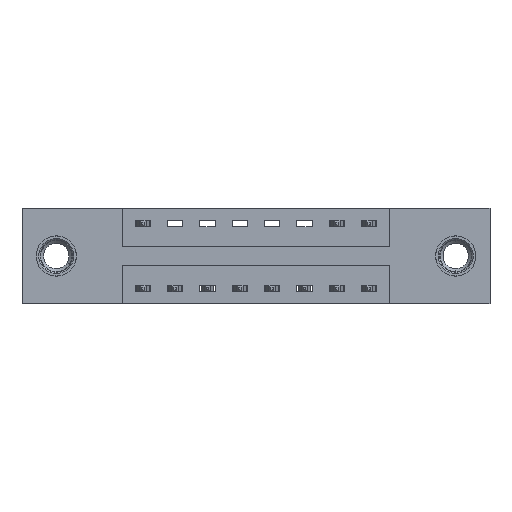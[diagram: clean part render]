
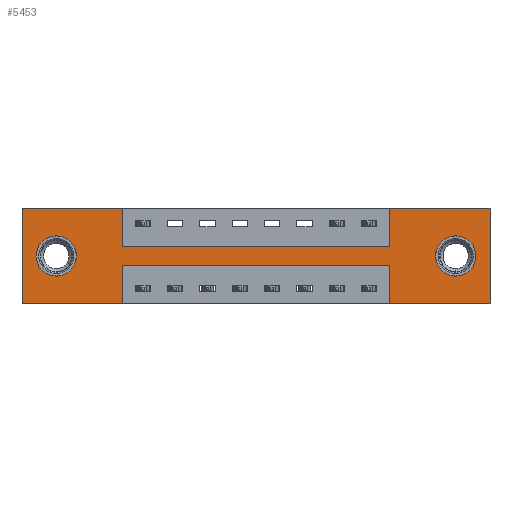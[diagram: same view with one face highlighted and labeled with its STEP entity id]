
A CAD part, front view. The second image highlights one B-rep face of the part: STEP entity #5453.
In plain terms, the highlighted planar face has unit normal (0, -1, 0).
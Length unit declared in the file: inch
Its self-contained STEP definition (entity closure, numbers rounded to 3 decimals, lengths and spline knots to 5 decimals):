
#43 = DIRECTION ( 'NONE',  ( 0., 0., 1. ) ) ;
#82 = VECTOR ( 'NONE', #8620, 39.37008 ) ;
#323 = EDGE_CURVE ( 'NONE', #2774, #729, #4343, .T. ) ;
#348 = CARTESIAN_POINT ( 'NONE',  ( 0., 0., 0. ) ) ;
#426 = DIRECTION ( 'NONE',  ( -1., 0., 0. ) ) ;
#499 = ORIENTED_EDGE ( 'NONE', *, *, #1237, .F. ) ;
#500 = CARTESIAN_POINT ( 'NONE',  ( 1.6775, 0., -0.107 ) ) ;
#535 = CARTESIAN_POINT ( 'NONE',  ( 0., 0., -0.37 ) ) ;
#729 = VERTEX_POINT ( 'NONE', #921 ) ;
#777 = VECTOR ( 'NONE', #8164, 39.37008 ) ;
#783 = ORIENTED_EDGE ( 'NONE', *, *, #1724, .F. ) ;
#921 = CARTESIAN_POINT ( 'NONE',  ( 0.3875, 0., -0.15 ) ) ;
#1048 = ORIENTED_EDGE ( 'NONE', *, *, #2806, .F. ) ;
#1144 = LINE ( 'NONE', #5271, #7589 ) ;
#1211 = DIRECTION ( 'NONE',  ( 0., 1., 0. ) ) ;
#1237 = EDGE_CURVE ( 'NONE', #1583, #8668, #10362, .T. ) ;
#1301 = EDGE_CURVE ( 'NONE', #6585, #1547, #5235, .T. ) ;
#1326 = ORIENTED_EDGE ( 'NONE', *, *, #1554, .F. ) ;
#1367 = CARTESIAN_POINT ( 'NONE',  ( 1.6775, 0., -0.263 ) ) ;
#1395 = CARTESIAN_POINT ( 'NONE',  ( 0.3875, 0., -0.37 ) ) ;
#1454 = CARTESIAN_POINT ( 'NONE',  ( 0., 0., 0. ) ) ;
#1469 = VERTEX_POINT ( 'NONE', #2483 ) ;
#1479 = VECTOR ( 'NONE', #8681, 39.37008 ) ;
#1481 = LINE ( 'NONE', #2366, #10096 ) ;
#1547 = VERTEX_POINT ( 'NONE', #500 ) ;
#1554 = EDGE_CURVE ( 'NONE', #8668, #8877, #9892, .T. ) ;
#1583 = VERTEX_POINT ( 'NONE', #5375 ) ;
#1646 = VERTEX_POINT ( 'NONE', #348 ) ;
#1655 = EDGE_CURVE ( 'NONE', #7522, #2655, #6432, .T. ) ;
#1724 = EDGE_CURVE ( 'NONE', #9123, #7522, #5678, .T. ) ;
#1829 = CARTESIAN_POINT ( 'NONE',  ( 0.1325, 0., -0.185 ) ) ;
#1849 = FACE_BOUND ( 'NONE', #3114, .T. ) ;
#1900 = CARTESIAN_POINT ( 'NONE',  ( 0.3875, 0., 0. ) ) ;
#1950 = CIRCLE ( 'NONE', #3902, 0.078 ) ;
#1995 = VERTEX_POINT ( 'NONE', #9253 ) ;
#2045 = VECTOR ( 'NONE', #6008, 39.37008 ) ;
#2064 = EDGE_CURVE ( 'NONE', #1646, #2774, #6168, .T. ) ;
#2086 = CIRCLE ( 'NONE', #3542, 0.078 ) ;
#2105 = DIRECTION ( 'NONE',  ( -1., 0., 0. ) ) ;
#2224 = DIRECTION ( 'NONE',  ( 0., 0., -1. ) ) ;
#2284 = ORIENTED_EDGE ( 'NONE', *, *, #10552, .T. ) ;
#2366 = CARTESIAN_POINT ( 'NONE',  ( 0., 0., 0. ) ) ;
#2483 = CARTESIAN_POINT ( 'NONE',  ( 0.1325, 0., -0.263 ) ) ;
#2561 = ORIENTED_EDGE ( 'NONE', *, *, #10851, .T. ) ;
#2655 = VERTEX_POINT ( 'NONE', #7575 ) ;
#2706 = DIRECTION ( 'NONE',  ( 0., 0., 1. ) ) ;
#2774 = VERTEX_POINT ( 'NONE', #1900 ) ;
#2806 = EDGE_CURVE ( 'NONE', #729, #4766, #6403, .T. ) ;
#2838 = ORIENTED_EDGE ( 'NONE', *, *, #10377, .F. ) ;
#2917 = CARTESIAN_POINT ( 'NONE',  ( 1.81, 0., 0. ) ) ;
#3088 = EDGE_CURVE ( 'NONE', #8877, #1646, #1481, .T. ) ;
#3114 = EDGE_LOOP ( 'NONE', ( #2561, #4838 ) ) ;
#3122 = CARTESIAN_POINT ( 'NONE',  ( 1.81, 0., 0. ) ) ;
#3245 = DIRECTION ( 'NONE',  ( 0., 0., 1. ) ) ;
#3381 = ORIENTED_EDGE ( 'NONE', *, *, #323, .F. ) ;
#3455 = VERTEX_POINT ( 'NONE', #4528 ) ;
#3542 = AXIS2_PLACEMENT_3D ( 'NONE', #6314, #1211, #7133 ) ;
#3902 = AXIS2_PLACEMENT_3D ( 'NONE', #1829, #7675, #2706 ) ;
#3978 = EDGE_LOOP ( 'NONE', ( #499, #2838, #5094, #9453, #783, #7503, #9712, #1048, #3381, #7757, #9970, #1326 ) ) ;
#4111 = DIRECTION ( 'NONE',  ( 0., 0., 1. ) ) ;
#4220 = VECTOR ( 'NONE', #2105, 39.37008 ) ;
#4287 = LINE ( 'NONE', #9872, #8645 ) ;
#4343 = LINE ( 'NONE', #6040, #2045 ) ;
#4528 = CARTESIAN_POINT ( 'NONE',  ( 1.4225, 0., 0. ) ) ;
#4574 = ORIENTED_EDGE ( 'NONE', *, *, #1301, .T. ) ;
#4602 = EDGE_CURVE ( 'NONE', #3455, #9123, #5478, .T. ) ;
#4766 = VERTEX_POINT ( 'NONE', #9213 ) ;
#4838 = ORIENTED_EDGE ( 'NONE', *, *, #6191, .T. ) ;
#5078 = DIRECTION ( 'NONE',  ( 0., 0., -1. ) ) ;
#5094 = ORIENTED_EDGE ( 'NONE', *, *, #9754, .F. ) ;
#5235 = CIRCLE ( 'NONE', #9016, 0.078 ) ;
#5248 = DIRECTION ( 'NONE',  ( 0., 1., 0. ) ) ;
#5271 = CARTESIAN_POINT ( 'NONE',  ( 0.3875, 0., -0.22 ) ) ;
#5375 = CARTESIAN_POINT ( 'NONE',  ( 0.3875, 0., -0.22 ) ) ;
#5453 = ADVANCED_FACE ( 'NONE', ( #8780, #1849, #8509 ), #7485, .T. ) ;
#5478 = LINE ( 'NONE', #1454, #777 ) ;
#5613 = DIRECTION ( 'NONE',  ( 0., 0., -1. ) ) ;
#5678 = LINE ( 'NONE', #3122, #7303 ) ;
#5731 = DIRECTION ( 'NONE',  ( 0., 1., 0. ) ) ;
#5734 = VERTEX_POINT ( 'NONE', #9595 ) ;
#5800 = CARTESIAN_POINT ( 'NONE',  ( 1.6775, 0., -0.185 ) ) ;
#5921 = VECTOR ( 'NONE', #10187, 39.37008 ) ;
#6008 = DIRECTION ( 'NONE',  ( 0., 0., -1. ) ) ;
#6040 = CARTESIAN_POINT ( 'NONE',  ( 0.3875, 0., 0. ) ) ;
#6168 = LINE ( 'NONE', #8486, #5921 ) ;
#6191 = EDGE_CURVE ( 'NONE', #1469, #5734, #7233, .T. ) ;
#6236 = VECTOR ( 'NONE', #6268, 39.37008 ) ;
#6268 = DIRECTION ( 'NONE',  ( 0., 0., 1. ) ) ;
#6314 = CARTESIAN_POINT ( 'NONE',  ( 1.6775, 0., -0.185 ) ) ;
#6403 = LINE ( 'NONE', #7828, #82 ) ;
#6432 = LINE ( 'NONE', #7128, #4220 ) ;
#6585 = VERTEX_POINT ( 'NONE', #1367 ) ;
#6698 = CARTESIAN_POINT ( 'NONE',  ( 1.81, 0., -0.37 ) ) ;
#7128 = CARTESIAN_POINT ( 'NONE',  ( 0., 0., -0.37 ) ) ;
#7133 = DIRECTION ( 'NONE',  ( 0., 0., -1. ) ) ;
#7233 = CIRCLE ( 'NONE', #7516, 0.078 ) ;
#7303 = VECTOR ( 'NONE', #2224, 39.37008 ) ;
#7485 = PLANE ( 'NONE',  #10854 ) ;
#7503 = ORIENTED_EDGE ( 'NONE', *, *, #4602, .F. ) ;
#7516 = AXIS2_PLACEMENT_3D ( 'NONE', #10139, #5248, #43 ) ;
#7522 = VERTEX_POINT ( 'NONE', #6698 ) ;
#7575 = CARTESIAN_POINT ( 'NONE',  ( 1.4225, 0., -0.37 ) ) ;
#7589 = VECTOR ( 'NONE', #9382, 39.37008 ) ;
#7660 = CARTESIAN_POINT ( 'NONE',  ( 0., 0., -0.37 ) ) ;
#7675 = DIRECTION ( 'NONE',  ( 0., 1., 0. ) ) ;
#7678 = VECTOR ( 'NONE', #426, 39.37008 ) ;
#7757 = ORIENTED_EDGE ( 'NONE', *, *, #2064, .F. ) ;
#7828 = CARTESIAN_POINT ( 'NONE',  ( 0.3875, 0., -0.15 ) ) ;
#7903 = EDGE_LOOP ( 'NONE', ( #2284, #4574 ) ) ;
#8164 = DIRECTION ( 'NONE',  ( 1., 0., 0. ) ) ;
#8315 = CARTESIAN_POINT ( 'NONE',  ( 0., 0., -0.37 ) ) ;
#8486 = CARTESIAN_POINT ( 'NONE',  ( 0., 0., 0. ) ) ;
#8509 = FACE_OUTER_BOUND ( 'NONE', #3978, .T. ) ;
#8620 = DIRECTION ( 'NONE',  ( 1., 0., 0. ) ) ;
#8629 = CARTESIAN_POINT ( 'NONE',  ( 0.3875, 0., -0.37 ) ) ;
#8632 = LINE ( 'NONE', #9508, #6236 ) ;
#8645 = VECTOR ( 'NONE', #4111, 39.37008 ) ;
#8668 = VERTEX_POINT ( 'NONE', #1395 ) ;
#8681 = DIRECTION ( 'NONE',  ( 0., 0., -1. ) ) ;
#8780 = FACE_BOUND ( 'NONE', #7903, .T. ) ;
#8877 = VERTEX_POINT ( 'NONE', #7660 ) ;
#9016 = AXIS2_PLACEMENT_3D ( 'NONE', #5800, #5731, #5613 ) ;
#9123 = VERTEX_POINT ( 'NONE', #2917 ) ;
#9213 = CARTESIAN_POINT ( 'NONE',  ( 1.4225, 0., -0.15 ) ) ;
#9253 = CARTESIAN_POINT ( 'NONE',  ( 1.4225, 0., -0.22 ) ) ;
#9366 = EDGE_CURVE ( 'NONE', #4766, #3455, #4287, .T. ) ;
#9382 = DIRECTION ( 'NONE',  ( -1., 0., 0. ) ) ;
#9453 = ORIENTED_EDGE ( 'NONE', *, *, #1655, .F. ) ;
#9508 = CARTESIAN_POINT ( 'NONE',  ( 1.4225, 0., -0.37 ) ) ;
#9595 = CARTESIAN_POINT ( 'NONE',  ( 0.1325, 0., -0.107 ) ) ;
#9712 = ORIENTED_EDGE ( 'NONE', *, *, #9366, .F. ) ;
#9754 = EDGE_CURVE ( 'NONE', #2655, #1995, #8632, .T. ) ;
#9872 = CARTESIAN_POINT ( 'NONE',  ( 1.4225, 0., 0. ) ) ;
#9892 = LINE ( 'NONE', #535, #7678 ) ;
#9970 = ORIENTED_EDGE ( 'NONE', *, *, #3088, .F. ) ;
#9985 = DIRECTION ( 'NONE',  ( 0., -1., 0. ) ) ;
#10096 = VECTOR ( 'NONE', #3245, 39.37008 ) ;
#10139 = CARTESIAN_POINT ( 'NONE',  ( 0.1325, 0., -0.185 ) ) ;
#10187 = DIRECTION ( 'NONE',  ( 1., 0., 0. ) ) ;
#10362 = LINE ( 'NONE', #8629, #1479 ) ;
#10377 = EDGE_CURVE ( 'NONE', #1995, #1583, #1144, .T. ) ;
#10552 = EDGE_CURVE ( 'NONE', #1547, #6585, #2086, .T. ) ;
#10851 = EDGE_CURVE ( 'NONE', #5734, #1469, #1950, .T. ) ;
#10854 = AXIS2_PLACEMENT_3D ( 'NONE', #8315, #9985, #5078 ) ;
